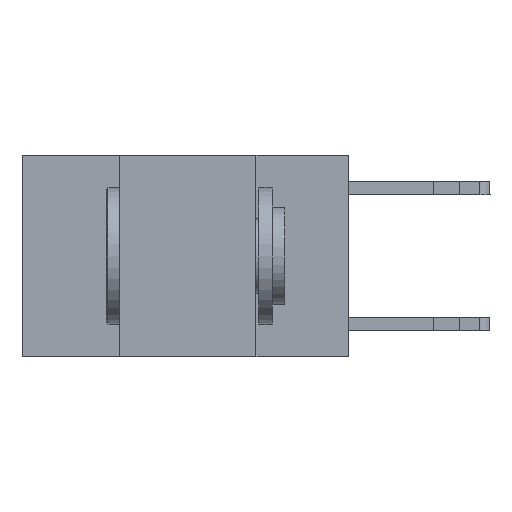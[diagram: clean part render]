
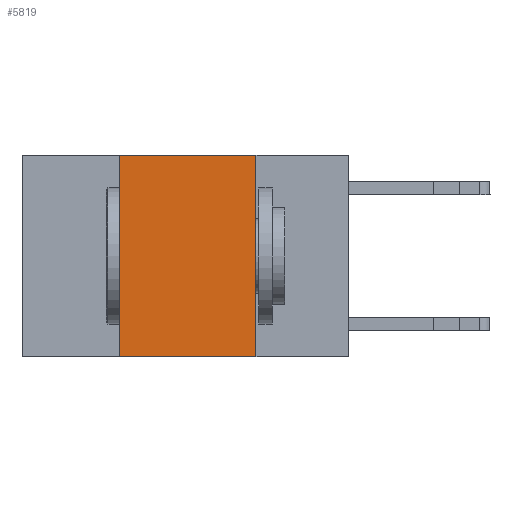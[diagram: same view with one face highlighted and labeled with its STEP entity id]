
A CAD part, left-side view. The second image highlights one B-rep face of the part: STEP entity #5819.
In plain terms, the highlighted planar face has unit normal (-1, 0, 0).
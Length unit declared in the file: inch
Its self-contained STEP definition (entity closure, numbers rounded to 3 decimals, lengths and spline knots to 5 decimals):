
#737 = CARTESIAN_POINT ( 'NONE',  ( 0., 0.17, -0.37 ) ) ;
#1065 = FACE_OUTER_BOUND ( 'NONE', #5397, .T. ) ;
#1388 = ORIENTED_EDGE ( 'NONE', *, *, #2374, .T. ) ;
#1767 = VERTEX_POINT ( 'NONE', #13457 ) ;
#2121 = CARTESIAN_POINT ( 'NONE',  ( 0., 0.17, 0. ) ) ;
#2374 = EDGE_CURVE ( 'NONE', #1767, #11881, #5778, .T. ) ;
#2529 = CARTESIAN_POINT ( 'NONE',  ( 0., 0.6, 0. ) ) ;
#2818 = DIRECTION ( 'NONE',  ( 0., 0., -1. ) ) ;
#3272 = PLANE ( 'NONE',  #9959 ) ;
#4196 = VERTEX_POINT ( 'NONE', #2121 ) ;
#4419 = CARTESIAN_POINT ( 'NONE',  ( 0., 0.6, -0.37 ) ) ;
#4463 = CARTESIAN_POINT ( 'NONE',  ( 0., 0.6, 0. ) ) ;
#4733 = VECTOR ( 'NONE', #4856, 39.37008 ) ;
#4817 = CARTESIAN_POINT ( 'NONE',  ( 0., 0.42, 0. ) ) ;
#4856 = DIRECTION ( 'NONE',  ( 0., -1., 0. ) ) ;
#5397 = EDGE_LOOP ( 'NONE', ( #8023, #5945, #12576, #1388 ) ) ;
#5778 = LINE ( 'NONE', #4419, #6089 ) ;
#5819 = ADVANCED_FACE ( 'NONE', ( #1065 ), #3272, .F. ) ;
#5945 = ORIENTED_EDGE ( 'NONE', *, *, #10338, .F. ) ;
#5983 = DIRECTION ( 'NONE',  ( 1., 0., 0. ) ) ;
#6089 = VECTOR ( 'NONE', #6976, 39.37008 ) ;
#6840 = LINE ( 'NONE', #12703, #7059 ) ;
#6976 = DIRECTION ( 'NONE',  ( 0., -1., 0. ) ) ;
#7059 = VECTOR ( 'NONE', #2818, 39.37008 ) ;
#7811 = VERTEX_POINT ( 'NONE', #14640 ) ;
#8023 = ORIENTED_EDGE ( 'NONE', *, *, #11959, .F. ) ;
#9959 = AXIS2_PLACEMENT_3D ( 'NONE', #4463, #5983, #11967 ) ;
#10338 = EDGE_CURVE ( 'NONE', #7811, #4196, #14496, .T. ) ;
#11183 = EDGE_CURVE ( 'NONE', #1767, #7811, #12932, .T. ) ;
#11881 = VERTEX_POINT ( 'NONE', #737 ) ;
#11959 = EDGE_CURVE ( 'NONE', #4196, #11881, #6840, .T. ) ;
#11967 = DIRECTION ( 'NONE',  ( 0., 0., -1. ) ) ;
#12576 = ORIENTED_EDGE ( 'NONE', *, *, #11183, .F. ) ;
#12703 = CARTESIAN_POINT ( 'NONE',  ( 0., 0.17, 0. ) ) ;
#12932 = LINE ( 'NONE', #4817, #13564 ) ;
#13169 = DIRECTION ( 'NONE',  ( 0., 0., 1. ) ) ;
#13457 = CARTESIAN_POINT ( 'NONE',  ( 0., 0.42, -0.37 ) ) ;
#13564 = VECTOR ( 'NONE', #13169, 39.37008 ) ;
#14496 = LINE ( 'NONE', #2529, #4733 ) ;
#14640 = CARTESIAN_POINT ( 'NONE',  ( 0., 0.42, 0. ) ) ;
